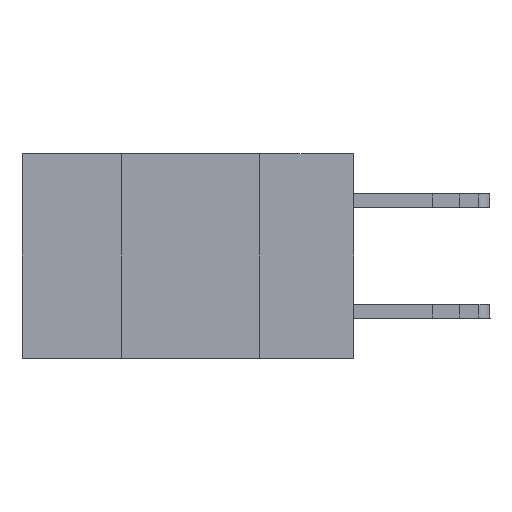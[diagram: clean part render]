
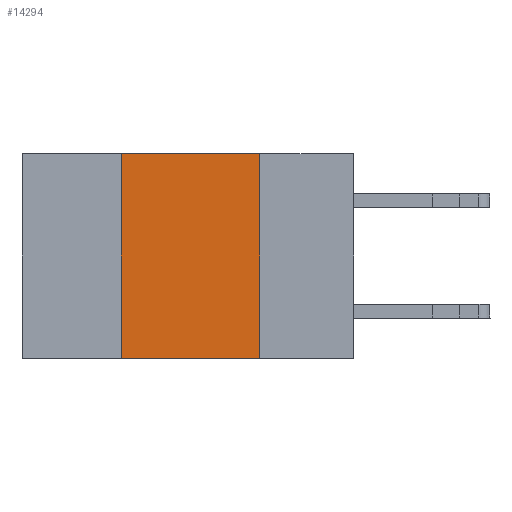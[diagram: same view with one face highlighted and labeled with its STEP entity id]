
A CAD part, left-side view. The second image highlights one B-rep face of the part: STEP entity #14294.
In plain terms, the highlighted planar face has unit normal (-1, 0, 0).
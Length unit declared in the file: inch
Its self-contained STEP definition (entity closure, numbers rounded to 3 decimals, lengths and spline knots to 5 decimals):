
#744 = EDGE_CURVE ( 'NONE', #13195, #15974, #4718, .T. ) ;
#792 = CARTESIAN_POINT ( 'NONE',  ( 0., 0.6, -0.37 ) ) ;
#1181 = EDGE_CURVE ( 'NONE', #19588, #14229, #17668, .T. ) ;
#2237 = ORIENTED_EDGE ( 'NONE', *, *, #14150, .T. ) ;
#2389 = EDGE_LOOP ( 'NONE', ( #21035, #9472, #11430, #2237 ) ) ;
#3300 = LINE ( 'NONE', #4779, #15712 ) ;
#3913 = VECTOR ( 'NONE', #6612, 39.37008 ) ;
#4718 = LINE ( 'NONE', #12291, #9816 ) ;
#4779 = CARTESIAN_POINT ( 'NONE',  ( 0., 0.6, 0. ) ) ;
#5752 = DIRECTION ( 'NONE',  ( 1., 0., 0. ) ) ;
#6612 = DIRECTION ( 'NONE',  ( 0., 0., 1. ) ) ;
#6716 = CARTESIAN_POINT ( 'NONE',  ( 0., 0.17, -0.37 ) ) ;
#9472 = ORIENTED_EDGE ( 'NONE', *, *, #15647, .F. ) ;
#9714 = CARTESIAN_POINT ( 'NONE',  ( 0., 0.6, 0. ) ) ;
#9816 = VECTOR ( 'NONE', #23394, 39.37008 ) ;
#10340 = DIRECTION ( 'NONE',  ( 0., -1., 0. ) ) ;
#10937 = CARTESIAN_POINT ( 'NONE',  ( 0., 0.42, 0. ) ) ;
#11430 = ORIENTED_EDGE ( 'NONE', *, *, #1181, .F. ) ;
#12291 = CARTESIAN_POINT ( 'NONE',  ( 0., 0.17, 0. ) ) ;
#13070 = FACE_OUTER_BOUND ( 'NONE', #2389, .T. ) ;
#13195 = VERTEX_POINT ( 'NONE', #14777 ) ;
#13556 = CARTESIAN_POINT ( 'NONE',  ( 0., 0.42, -0.37 ) ) ;
#14068 = LINE ( 'NONE', #792, #17952 ) ;
#14150 = EDGE_CURVE ( 'NONE', #19588, #15974, #14068, .T. ) ;
#14229 = VERTEX_POINT ( 'NONE', #10937 ) ;
#14294 = ADVANCED_FACE ( 'NONE', ( #13070 ), #24427, .F. ) ;
#14777 = CARTESIAN_POINT ( 'NONE',  ( 0., 0.17, 0. ) ) ;
#15647 = EDGE_CURVE ( 'NONE', #14229, #13195, #3300, .T. ) ;
#15712 = VECTOR ( 'NONE', #20138, 39.37008 ) ;
#15974 = VERTEX_POINT ( 'NONE', #6716 ) ;
#16075 = CARTESIAN_POINT ( 'NONE',  ( 0., 0.42, 0. ) ) ;
#17668 = LINE ( 'NONE', #16075, #3913 ) ;
#17952 = VECTOR ( 'NONE', #10340, 39.37008 ) ;
#19588 = VERTEX_POINT ( 'NONE', #13556 ) ;
#20138 = DIRECTION ( 'NONE',  ( 0., -1., 0. ) ) ;
#20717 = DIRECTION ( 'NONE',  ( 0., 0., -1. ) ) ;
#21035 = ORIENTED_EDGE ( 'NONE', *, *, #744, .F. ) ;
#21843 = AXIS2_PLACEMENT_3D ( 'NONE', #9714, #5752, #20717 ) ;
#23394 = DIRECTION ( 'NONE',  ( 0., 0., -1. ) ) ;
#24427 = PLANE ( 'NONE',  #21843 ) ;
